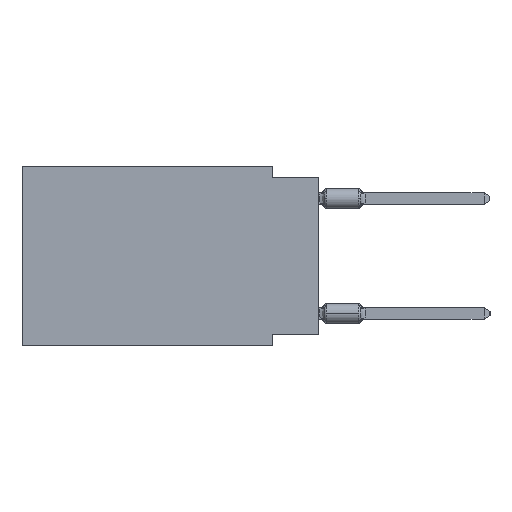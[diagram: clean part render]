
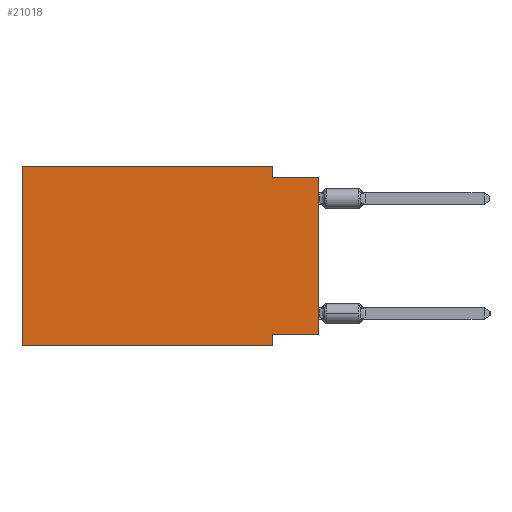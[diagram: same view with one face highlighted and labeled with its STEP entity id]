
A CAD part, left-side view. The second image highlights one B-rep face of the part: STEP entity #21018.
In plain terms, the highlighted planar face has unit normal (-1, 0, 0).
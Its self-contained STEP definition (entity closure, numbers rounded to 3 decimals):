
#99 = CARTESIAN_POINT ( 'NONE',  ( 0., 2.54, -9.906 ) ) ;
#294 = AXIS2_PLACEMENT_3D ( 'NONE', #36247, #40909, #8746 ) ;
#568 = ORIENTED_EDGE ( 'NONE', *, *, #49949, .T. ) ;
#1126 = VECTOR ( 'NONE', #16431, 1000. ) ;
#2399 = CARTESIAN_POINT ( 'NONE',  ( 0., 16.383, 0. ) ) ;
#2411 = LINE ( 'NONE', #34283, #1126 ) ;
#2978 = CARTESIAN_POINT ( 'NONE',  ( 0., 2.54, 0. ) ) ;
#4364 = LINE ( 'NONE', #22222, #19433 ) ;
#4854 = VERTEX_POINT ( 'NONE', #16523 ) ;
#4947 = PLANE ( 'NONE',  #294 ) ;
#5512 = VECTOR ( 'NONE', #53951, 1000. ) ;
#6150 = ORIENTED_EDGE ( 'NONE', *, *, #10598, .F. ) ;
#7063 = LINE ( 'NONE', #12844, #33645 ) ;
#8746 = DIRECTION ( 'NONE',  ( 0., 0., -1. ) ) ;
#10017 = ORIENTED_EDGE ( 'NONE', *, *, #19237, .F. ) ;
#10598 = EDGE_CURVE ( 'NONE', #37369, #19568, #2411, .T. ) ;
#11389 = CARTESIAN_POINT ( 'NONE',  ( 0., 16.383, 0. ) ) ;
#12244 = ORIENTED_EDGE ( 'NONE', *, *, #38387, .F. ) ;
#12844 = CARTESIAN_POINT ( 'NONE',  ( 0., 0., -9.271 ) ) ;
#12850 = LINE ( 'NONE', #15853, #49328 ) ;
#14773 = EDGE_CURVE ( 'NONE', #18821, #51300, #12850, .T. ) ;
#14896 = EDGE_CURVE ( 'NONE', #18821, #15350, #4364, .T. ) ;
#14951 = VECTOR ( 'NONE', #41892, 1000. ) ;
#15350 = VERTEX_POINT ( 'NONE', #18908 ) ;
#15401 = LINE ( 'NONE', #33240, #51189 ) ;
#15853 = CARTESIAN_POINT ( 'NONE',  ( 0., 16.383, 0. ) ) ;
#16431 = DIRECTION ( 'NONE',  ( 0., 0., -1. ) ) ;
#16523 = CARTESIAN_POINT ( 'NONE',  ( 0., 2.54, -9.271 ) ) ;
#18821 = VERTEX_POINT ( 'NONE', #51872 ) ;
#18908 = CARTESIAN_POINT ( 'NONE',  ( 0., 2.54, -9.906 ) ) ;
#19037 = VERTEX_POINT ( 'NONE', #24071 ) ;
#19053 = EDGE_CURVE ( 'NONE', #51300, #37369, #28455, .T. ) ;
#19237 = EDGE_CURVE ( 'NONE', #25217, #4854, #7063, .T. ) ;
#19433 = VECTOR ( 'NONE', #40051, 1000. ) ;
#19568 = VERTEX_POINT ( 'NONE', #37941 ) ;
#20657 = VECTOR ( 'NONE', #35778, 1000. ) ;
#21018 = ADVANCED_FACE ( 'NONE', ( #27191 ), #4947, .F. ) ;
#22222 = CARTESIAN_POINT ( 'NONE',  ( 0., 16.383, -9.906 ) ) ;
#23537 = LINE ( 'NONE', #45470, #5512 ) ;
#24071 = CARTESIAN_POINT ( 'NONE',  ( 0., 0., -0.635 ) ) ;
#25102 = CARTESIAN_POINT ( 'NONE',  ( 0., 0., -9.271 ) ) ;
#25217 = VERTEX_POINT ( 'NONE', #25102 ) ;
#27191 = FACE_OUTER_BOUND ( 'NONE', #57404, .T. ) ;
#28455 = LINE ( 'NONE', #2399, #14951 ) ;
#33240 = CARTESIAN_POINT ( 'NONE',  ( 0., 0., 0. ) ) ;
#33645 = VECTOR ( 'NONE', #40040, 1000. ) ;
#33699 = DIRECTION ( 'NONE',  ( 0., 0., 1. ) ) ;
#34283 = CARTESIAN_POINT ( 'NONE',  ( 0., 2.54, 0. ) ) ;
#34606 = LINE ( 'NONE', #99, #20657 ) ;
#35778 = DIRECTION ( 'NONE',  ( 0., 0., -1. ) ) ;
#36247 = CARTESIAN_POINT ( 'NONE',  ( 0., 16.383, 0. ) ) ;
#37369 = VERTEX_POINT ( 'NONE', #2978 ) ;
#37941 = CARTESIAN_POINT ( 'NONE',  ( 0., 2.54, -0.635 ) ) ;
#38387 = EDGE_CURVE ( 'NONE', #19568, #19037, #23537, .T. ) ;
#40040 = DIRECTION ( 'NONE',  ( 0., 1., 0. ) ) ;
#40051 = DIRECTION ( 'NONE',  ( 0., -1., 0. ) ) ;
#40909 = DIRECTION ( 'NONE',  ( 1., 0., 0. ) ) ;
#41200 = EDGE_CURVE ( 'NONE', #4854, #15350, #34606, .T. ) ;
#41892 = DIRECTION ( 'NONE',  ( 0., -1., 0. ) ) ;
#44445 = ORIENTED_EDGE ( 'NONE', *, *, #14896, .T. ) ;
#45470 = CARTESIAN_POINT ( 'NONE',  ( 0., 0., -0.635 ) ) ;
#48275 = ORIENTED_EDGE ( 'NONE', *, *, #14773, .F. ) ;
#49328 = VECTOR ( 'NONE', #33699, 1000. ) ;
#49949 = EDGE_CURVE ( 'NONE', #25217, #19037, #15401, .T. ) ;
#51073 = DIRECTION ( 'NONE',  ( 0., 0., 1. ) ) ;
#51189 = VECTOR ( 'NONE', #51073, 1000. ) ;
#51300 = VERTEX_POINT ( 'NONE', #11389 ) ;
#51872 = CARTESIAN_POINT ( 'NONE',  ( 0., 16.383, -9.906 ) ) ;
#53755 = ORIENTED_EDGE ( 'NONE', *, *, #19053, .F. ) ;
#53951 = DIRECTION ( 'NONE',  ( 0., -1., 0. ) ) ;
#54211 = ORIENTED_EDGE ( 'NONE', *, *, #41200, .F. ) ;
#57404 = EDGE_LOOP ( 'NONE', ( #568, #12244, #6150, #53755, #48275, #44445, #54211, #10017 ) ) ;
